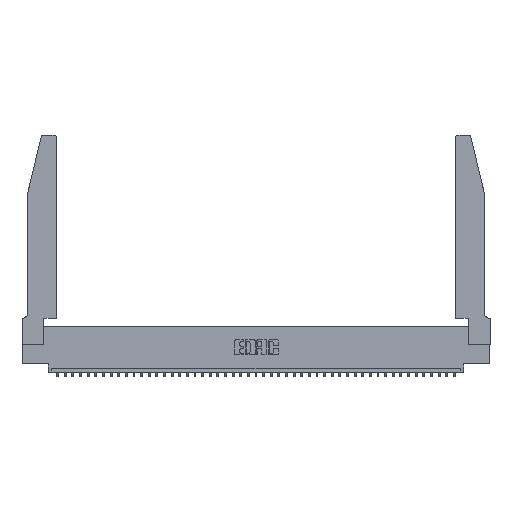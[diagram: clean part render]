
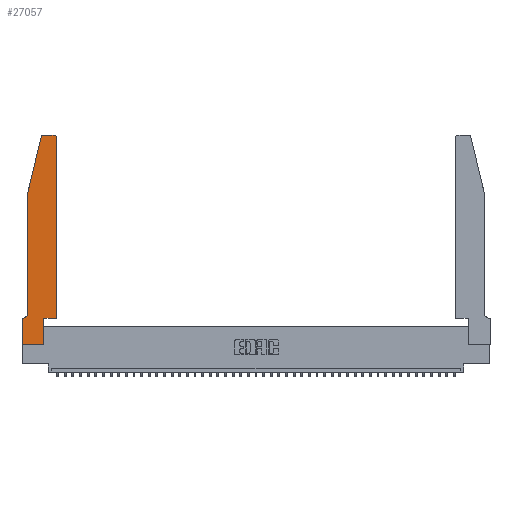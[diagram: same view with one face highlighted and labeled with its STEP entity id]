
A CAD part, top view. The second image highlights one B-rep face of the part: STEP entity #27057.
In plain terms, the highlighted planar face has unit normal (0, 0, 1).
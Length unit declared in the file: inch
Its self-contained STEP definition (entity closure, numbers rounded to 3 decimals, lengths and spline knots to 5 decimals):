
#70 = CIRCLE ( 'NONE', #31582, 0.03 ) ;
#696 = CARTESIAN_POINT ( 'NONE',  ( 0.4205, 2.75, 0.37 ) ) ;
#1161 = CARTESIAN_POINT ( 'NONE',  ( 0.2865, 0.35, 0.37 ) ) ;
#1266 = EDGE_CURVE ( 'NONE', #30253, #16695, #22989, .T. ) ;
#2279 = DIRECTION ( 'NONE',  ( -1., 0., 0. ) ) ;
#2945 = DIRECTION ( 'NONE',  ( 0., 0., 1. ) ) ;
#3090 = ORIENTED_EDGE ( 'NONE', *, *, #27708, .T. ) ;
#3208 = CIRCLE ( 'NONE', #12914, 0.07 ) ;
#3325 = ORIENTED_EDGE ( 'NONE', *, *, #1266, .T. ) ;
#6021 = CARTESIAN_POINT ( 'NONE',  ( 0., 0., 0.37 ) ) ;
#7384 = CARTESIAN_POINT ( 'NONE',  ( 0.4505, 0.35, 0.37 ) ) ;
#7425 = DIRECTION ( 'NONE',  ( 0., -1., 0. ) ) ;
#8027 = ORIENTED_EDGE ( 'NONE', *, *, #40189, .T. ) ;
#8156 = FACE_OUTER_BOUND ( 'NONE', #19482, .T. ) ;
#9249 = CARTESIAN_POINT ( 'NONE',  ( 0.0755, 2., 0.37 ) ) ;
#9397 = LINE ( 'NONE', #7384, #11499 ) ;
#10274 = VERTEX_POINT ( 'NONE', #20530 ) ;
#10776 = VECTOR ( 'NONE', #41291, 39.37008 ) ;
#11427 = DIRECTION ( 'NONE',  ( -1., 0., 0. ) ) ;
#11499 = VECTOR ( 'NONE', #20544, 39.37008 ) ;
#11697 = ORIENTED_EDGE ( 'NONE', *, *, #39750, .T. ) ;
#12319 = VECTOR ( 'NONE', #7425, 39.37008 ) ;
#12914 = AXIS2_PLACEMENT_3D ( 'NONE', #34801, #30991, #11427 ) ;
#13967 = CARTESIAN_POINT ( 'NONE',  ( 0., 0., 0.37 ) ) ;
#14055 = PLANE ( 'NONE',  #19574 ) ;
#14094 = VECTOR ( 'NONE', #35051, 39.37008 ) ;
#14884 = VERTEX_POINT ( 'NONE', #39486 ) ;
#15157 = ORIENTED_EDGE ( 'NONE', *, *, #27866, .T. ) ;
#15524 = CARTESIAN_POINT ( 'NONE',  ( 0.0755, 0.42, 0.37 ) ) ;
#16328 = AXIS2_PLACEMENT_3D ( 'NONE', #39653, #2945, #29662 ) ;
#16695 = VERTEX_POINT ( 'NONE', #28232 ) ;
#16909 = ORIENTED_EDGE ( 'NONE', *, *, #26054, .T. ) ;
#17248 = VERTEX_POINT ( 'NONE', #9249 ) ;
#17830 = DIRECTION ( 'NONE',  ( 0., 0., 1. ) ) ;
#18063 = LINE ( 'NONE', #38854, #24850 ) ;
#18619 = VERTEX_POINT ( 'NONE', #696 ) ;
#19430 = LINE ( 'NONE', #35611, #36233 ) ;
#19482 = EDGE_LOOP ( 'NONE', ( #33127, #3325, #11697, #36484, #3090, #16909, #8027, #43277, #15157, #41518, #30550, #34628 ) ) ;
#19574 = AXIS2_PLACEMENT_3D ( 'NONE', #24383, #17830, #40965 ) ;
#19873 = VECTOR ( 'NONE', #41725, 39.37008 ) ;
#19926 = CARTESIAN_POINT ( 'NONE',  ( 0., 0.35, 0.37 ) ) ;
#20530 = CARTESIAN_POINT ( 'NONE',  ( 0.2865, 0.35, 0.37 ) ) ;
#20544 = DIRECTION ( 'NONE',  ( 1., 0., 0. ) ) ;
#20796 = CARTESIAN_POINT ( 'NONE',  ( 0.2865, 0., 0.37 ) ) ;
#20857 = VERTEX_POINT ( 'NONE', #15524 ) ;
#21589 = VECTOR ( 'NONE', #40195, 39.37008 ) ;
#22009 = LINE ( 'NONE', #6021, #30862 ) ;
#22989 = CIRCLE ( 'NONE', #16328, 0.03 ) ;
#23165 = CARTESIAN_POINT ( 'NONE',  ( 0.4505, 0.35, 0.37 ) ) ;
#24318 = EDGE_CURVE ( 'NONE', #24469, #26643, #18063, .T. ) ;
#24383 = CARTESIAN_POINT ( 'NONE',  ( 0., 0.35, 0.37 ) ) ;
#24469 = VERTEX_POINT ( 'NONE', #23165 ) ;
#24850 = VECTOR ( 'NONE', #25228, 39.37008 ) ;
#24999 = DIRECTION ( 'NONE',  ( 1., 0., 0. ) ) ;
#25228 = DIRECTION ( 'NONE',  ( 0., 1., 0. ) ) ;
#25712 = EDGE_CURVE ( 'NONE', #18619, #30253, #33618, .T. ) ;
#26054 = EDGE_CURVE ( 'NONE', #14884, #26356, #19430, .T. ) ;
#26057 = DIRECTION ( 'NONE',  ( 1., 0., 0. ) ) ;
#26356 = VERTEX_POINT ( 'NONE', #19926 ) ;
#26634 = LINE ( 'NONE', #38281, #14094 ) ;
#26643 = VERTEX_POINT ( 'NONE', #30851 ) ;
#27057 = ADVANCED_FACE ( 'NONE', ( #8156 ), #14055, .T. ) ;
#27708 = EDGE_CURVE ( 'NONE', #20857, #14884, #3208, .T. ) ;
#27866 = EDGE_CURVE ( 'NONE', #30099, #10274, #28739, .T. ) ;
#28232 = CARTESIAN_POINT ( 'NONE',  ( 0.25487, 2.72718, 0.37 ) ) ;
#28394 = EDGE_CURVE ( 'NONE', #10274, #24469, #9397, .T. ) ;
#28515 = EDGE_CURVE ( 'NONE', #17248, #20857, #26634, .T. ) ;
#28739 = LINE ( 'NONE', #1161, #19873 ) ;
#29662 = DIRECTION ( 'NONE',  ( 1., 0., 0. ) ) ;
#30099 = VERTEX_POINT ( 'NONE', #20796 ) ;
#30253 = VERTEX_POINT ( 'NONE', #43156 ) ;
#30550 = ORIENTED_EDGE ( 'NONE', *, *, #24318, .T. ) ;
#30851 = CARTESIAN_POINT ( 'NONE',  ( 0.4505, 2.72, 0.37 ) ) ;
#30862 = VECTOR ( 'NONE', #26057, 39.37008 ) ;
#30991 = DIRECTION ( 'NONE',  ( 0., 0., -1. ) ) ;
#31582 = AXIS2_PLACEMENT_3D ( 'NONE', #38638, #34812, #24999 ) ;
#33127 = ORIENTED_EDGE ( 'NONE', *, *, #25712, .T. ) ;
#33618 = LINE ( 'NONE', #39781, #21589 ) ;
#34514 = CARTESIAN_POINT ( 'NONE',  ( 0.0755, 2., 0.37 ) ) ;
#34628 = ORIENTED_EDGE ( 'NONE', *, *, #42564, .T. ) ;
#34801 = CARTESIAN_POINT ( 'NONE',  ( 0.0055, 0.42, 0.37 ) ) ;
#34812 = DIRECTION ( 'NONE',  ( 0., 0., 1. ) ) ;
#35051 = DIRECTION ( 'NONE',  ( 0., -1., 0. ) ) ;
#35611 = CARTESIAN_POINT ( 'NONE',  ( 0.0755, 0.35, 0.37 ) ) ;
#35658 = EDGE_CURVE ( 'NONE', #36788, #30099, #22009, .T. ) ;
#35895 = LINE ( 'NONE', #34514, #10776 ) ;
#36233 = VECTOR ( 'NONE', #2279, 39.37008 ) ;
#36484 = ORIENTED_EDGE ( 'NONE', *, *, #28515, .T. ) ;
#36788 = VERTEX_POINT ( 'NONE', #13967 ) ;
#37577 = CARTESIAN_POINT ( 'NONE',  ( 0., 0., 0.37 ) ) ;
#37916 = LINE ( 'NONE', #37577, #12319 ) ;
#38281 = CARTESIAN_POINT ( 'NONE',  ( 0.0755, 2., 0.37 ) ) ;
#38638 = CARTESIAN_POINT ( 'NONE',  ( 0.4205, 2.72, 0.37 ) ) ;
#38854 = CARTESIAN_POINT ( 'NONE',  ( 0.4505, 0.35, 0.37 ) ) ;
#39486 = CARTESIAN_POINT ( 'NONE',  ( 0.0055, 0.35, 0.37 ) ) ;
#39653 = CARTESIAN_POINT ( 'NONE',  ( 0.284, 2.72, 0.37 ) ) ;
#39750 = EDGE_CURVE ( 'NONE', #16695, #17248, #35895, .T. ) ;
#39781 = CARTESIAN_POINT ( 'NONE',  ( 0.2605, 2.75, 0.37 ) ) ;
#40189 = EDGE_CURVE ( 'NONE', #26356, #36788, #37916, .T. ) ;
#40195 = DIRECTION ( 'NONE',  ( -1., 0., 0. ) ) ;
#40965 = DIRECTION ( 'NONE',  ( 1., 0., 0. ) ) ;
#41291 = DIRECTION ( 'NONE',  ( -0.239, -0.971, 0. ) ) ;
#41518 = ORIENTED_EDGE ( 'NONE', *, *, #28394, .T. ) ;
#41725 = DIRECTION ( 'NONE',  ( 0., 1., 0. ) ) ;
#42564 = EDGE_CURVE ( 'NONE', #26643, #18619, #70, .T. ) ;
#43156 = CARTESIAN_POINT ( 'NONE',  ( 0.284, 2.75, 0.37 ) ) ;
#43277 = ORIENTED_EDGE ( 'NONE', *, *, #35658, .T. ) ;
